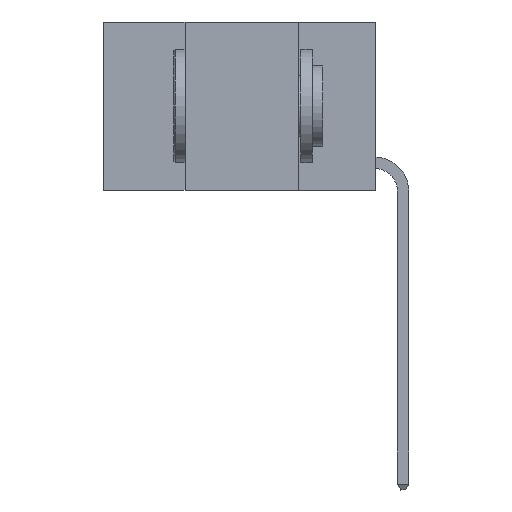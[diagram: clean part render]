
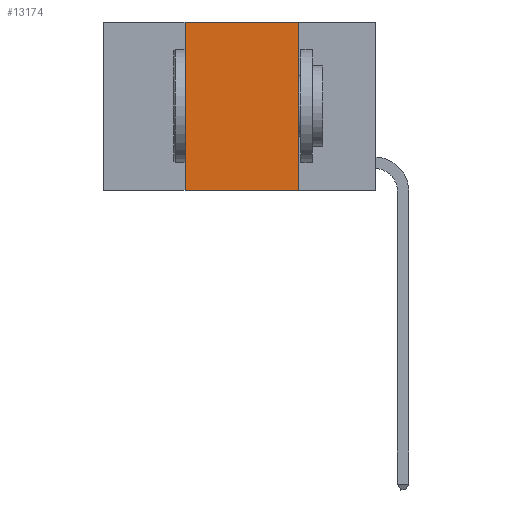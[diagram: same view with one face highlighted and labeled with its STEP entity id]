
A CAD part, left-side view. The second image highlights one B-rep face of the part: STEP entity #13174.
In plain terms, the highlighted planar face has unit normal (-1, 0, 0).
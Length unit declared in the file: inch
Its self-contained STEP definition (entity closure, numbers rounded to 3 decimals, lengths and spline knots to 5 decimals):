
#828 = DIRECTION ( 'NONE',  ( 0., 0., -1. ) ) ;
#1000 = CARTESIAN_POINT ( 'NONE',  ( 0., 0.17, -0.37 ) ) ;
#1014 = PLANE ( 'NONE',  #9768 ) ;
#2428 = CARTESIAN_POINT ( 'NONE',  ( 0., 0.6, 0. ) ) ;
#2519 = FACE_OUTER_BOUND ( 'NONE', #13337, .T. ) ;
#4106 = ORIENTED_EDGE ( 'NONE', *, *, #15551, .F. ) ;
#5145 = CARTESIAN_POINT ( 'NONE',  ( 0., 0.42, 0. ) ) ;
#5158 = CARTESIAN_POINT ( 'NONE',  ( 0., 0.42, 0. ) ) ;
#5625 = VECTOR ( 'NONE', #6583, 39.37008 ) ;
#6190 = VERTEX_POINT ( 'NONE', #15204 ) ;
#6583 = DIRECTION ( 'NONE',  ( 0., 0., 1. ) ) ;
#6910 = VERTEX_POINT ( 'NONE', #1000 ) ;
#7033 = ORIENTED_EDGE ( 'NONE', *, *, #11857, .F. ) ;
#7087 = CARTESIAN_POINT ( 'NONE',  ( 0., 0.6, 0. ) ) ;
#7694 = ORIENTED_EDGE ( 'NONE', *, *, #9249, .F. ) ;
#7890 = LINE ( 'NONE', #16839, #17377 ) ;
#8179 = DIRECTION ( 'NONE',  ( 1., 0., 0. ) ) ;
#8594 = ORIENTED_EDGE ( 'NONE', *, *, #11760, .T. ) ;
#9249 = EDGE_CURVE ( 'NONE', #13554, #11439, #12826, .T. ) ;
#9768 = AXIS2_PLACEMENT_3D ( 'NONE', #2428, #8179, #16841 ) ;
#10082 = DIRECTION ( 'NONE',  ( 0., -1., 0. ) ) ;
#11439 = VERTEX_POINT ( 'NONE', #13762 ) ;
#11760 = EDGE_CURVE ( 'NONE', #6190, #6910, #18258, .T. ) ;
#11857 = EDGE_CURVE ( 'NONE', #11439, #6910, #7890, .T. ) ;
#12547 = VECTOR ( 'NONE', #17974, 39.37008 ) ;
#12826 = LINE ( 'NONE', #7087, #12996 ) ;
#12996 = VECTOR ( 'NONE', #10082, 39.37008 ) ;
#13174 = ADVANCED_FACE ( 'NONE', ( #2519 ), #1014, .F. ) ;
#13337 = EDGE_LOOP ( 'NONE', ( #7033, #7694, #4106, #8594 ) ) ;
#13554 = VERTEX_POINT ( 'NONE', #5145 ) ;
#13762 = CARTESIAN_POINT ( 'NONE',  ( 0., 0.17, 0. ) ) ;
#14012 = LINE ( 'NONE', #5158, #5625 ) ;
#15204 = CARTESIAN_POINT ( 'NONE',  ( 0., 0.42, -0.37 ) ) ;
#15551 = EDGE_CURVE ( 'NONE', #6190, #13554, #14012, .T. ) ;
#16743 = CARTESIAN_POINT ( 'NONE',  ( 0., 0.6, -0.37 ) ) ;
#16839 = CARTESIAN_POINT ( 'NONE',  ( 0., 0.17, 0. ) ) ;
#16841 = DIRECTION ( 'NONE',  ( 0., 0., -1. ) ) ;
#17377 = VECTOR ( 'NONE', #828, 39.37008 ) ;
#17974 = DIRECTION ( 'NONE',  ( 0., -1., 0. ) ) ;
#18258 = LINE ( 'NONE', #16743, #12547 ) ;
